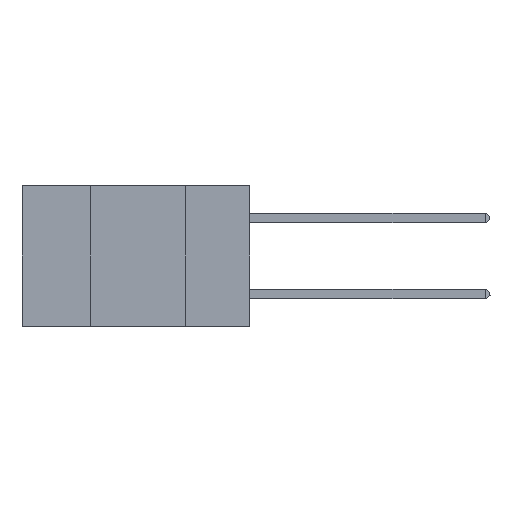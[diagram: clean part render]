
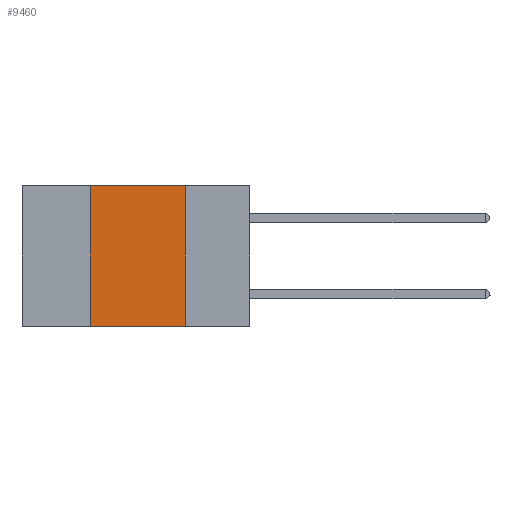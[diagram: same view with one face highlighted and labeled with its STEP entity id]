
A CAD part, left-side view. The second image highlights one B-rep face of the part: STEP entity #9460.
In plain terms, the highlighted planar face has unit normal (-1, 0, 0).
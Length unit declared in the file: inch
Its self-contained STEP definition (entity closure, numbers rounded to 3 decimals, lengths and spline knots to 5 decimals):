
#719 = FACE_OUTER_BOUND ( 'NONE', #10956, .T. ) ;
#779 = CARTESIAN_POINT ( 'NONE',  ( 0., 0.42, 0. ) ) ;
#1466 = PLANE ( 'NONE',  #10362 ) ;
#3050 = DIRECTION ( 'NONE',  ( 1., 0., 0. ) ) ;
#3249 = CARTESIAN_POINT ( 'NONE',  ( 0., 0.17, -0.37 ) ) ;
#3674 = EDGE_CURVE ( 'NONE', #13573, #16468, #11958, .T. ) ;
#4163 = CARTESIAN_POINT ( 'NONE',  ( 0., 0.6, 0. ) ) ;
#5176 = VERTEX_POINT ( 'NONE', #19846 ) ;
#5756 = ORIENTED_EDGE ( 'NONE', *, *, #15082, .F. ) ;
#5905 = DIRECTION ( 'NONE',  ( 0., 0., -1. ) ) ;
#5969 = LINE ( 'NONE', #4163, #18242 ) ;
#6589 = VECTOR ( 'NONE', #5905, 39.37008 ) ;
#7070 = EDGE_CURVE ( 'NONE', #5176, #16468, #15761, .T. ) ;
#8127 = ORIENTED_EDGE ( 'NONE', *, *, #11361, .F. ) ;
#9089 = CARTESIAN_POINT ( 'NONE',  ( 0., 0.6, 0. ) ) ;
#9460 = ADVANCED_FACE ( 'NONE', ( #719 ), #1466, .F. ) ;
#10362 = AXIS2_PLACEMENT_3D ( 'NONE', #9089, #3050, #12360 ) ;
#10418 = VECTOR ( 'NONE', #14014, 39.37008 ) ;
#10956 = EDGE_LOOP ( 'NONE', ( #13120, #5756, #8127, #12524 ) ) ;
#11361 = EDGE_CURVE ( 'NONE', #13573, #18653, #17604, .T. ) ;
#11380 = CARTESIAN_POINT ( 'NONE',  ( 0., 0.42, -0.37 ) ) ;
#11958 = LINE ( 'NONE', #15470, #15809 ) ;
#12219 = CARTESIAN_POINT ( 'NONE',  ( 0., 0.17, 0. ) ) ;
#12360 = DIRECTION ( 'NONE',  ( 0., 0., -1. ) ) ;
#12455 = DIRECTION ( 'NONE',  ( 0., -1., 0. ) ) ;
#12524 = ORIENTED_EDGE ( 'NONE', *, *, #3674, .T. ) ;
#13120 = ORIENTED_EDGE ( 'NONE', *, *, #7070, .F. ) ;
#13573 = VERTEX_POINT ( 'NONE', #11380 ) ;
#14014 = DIRECTION ( 'NONE',  ( 0., 0., 1. ) ) ;
#15082 = EDGE_CURVE ( 'NONE', #18653, #5176, #5969, .T. ) ;
#15470 = CARTESIAN_POINT ( 'NONE',  ( 0., 0.6, -0.37 ) ) ;
#15516 = CARTESIAN_POINT ( 'NONE',  ( 0., 0.42, 0. ) ) ;
#15761 = LINE ( 'NONE', #12219, #6589 ) ;
#15809 = VECTOR ( 'NONE', #18338, 39.37008 ) ;
#16468 = VERTEX_POINT ( 'NONE', #3249 ) ;
#17604 = LINE ( 'NONE', #15516, #10418 ) ;
#18242 = VECTOR ( 'NONE', #12455, 39.37008 ) ;
#18338 = DIRECTION ( 'NONE',  ( 0., -1., 0. ) ) ;
#18653 = VERTEX_POINT ( 'NONE', #779 ) ;
#19846 = CARTESIAN_POINT ( 'NONE',  ( 0., 0.17, 0. ) ) ;
